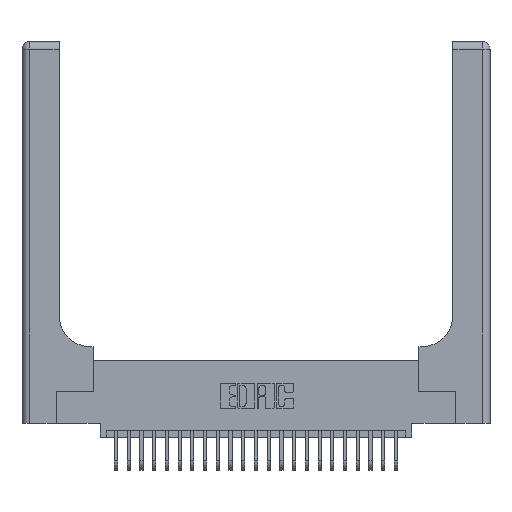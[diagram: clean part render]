
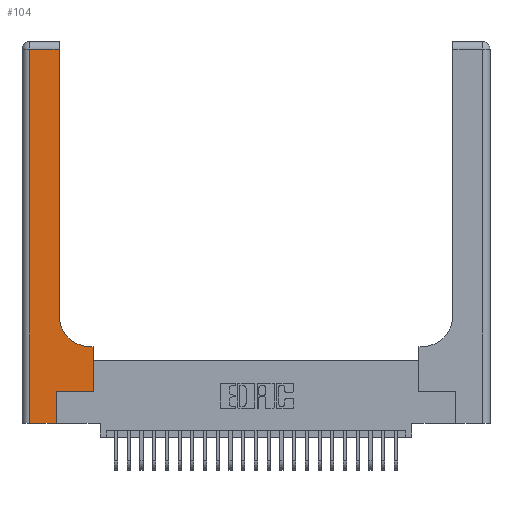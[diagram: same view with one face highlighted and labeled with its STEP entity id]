
A CAD part, top view. The second image highlights one B-rep face of the part: STEP entity #104.
In plain terms, the highlighted planar face has unit normal (0, 0, 1).
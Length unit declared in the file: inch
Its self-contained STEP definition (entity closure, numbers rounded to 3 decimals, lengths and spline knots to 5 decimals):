
#104 = ADVANCED_FACE ( 'NONE', ( #13858 ), #2259, .F. ) ;
#163 = AXIS2_PLACEMENT_3D ( 'NONE', #19622, #6866, #21750 ) ;
#419 = EDGE_CURVE ( 'NONE', #19018, #18135, #22831, .T. ) ;
#757 = ORIENTED_EDGE ( 'NONE', *, *, #15718, .T. ) ;
#1164 = DIRECTION ( 'NONE',  ( 1., 0., 0. ) ) ;
#1200 = EDGE_LOOP ( 'NONE', ( #757, #8010, #6784, #17955, #25926, #12365, #1759, #20742, #6190 ) ) ;
#1759 = ORIENTED_EDGE ( 'NONE', *, *, #11357, .T. ) ;
#1855 = EDGE_CURVE ( 'NONE', #12379, #5063, #2435, .T. ) ;
#2195 = DIRECTION ( 'NONE',  ( -1., 0., 0. ) ) ;
#2230 = DIRECTION ( 'NONE',  ( 0., 0., -1. ) ) ;
#2259 = PLANE ( 'NONE',  #24489 ) ;
#2435 = LINE ( 'NONE', #6089, #13146 ) ;
#2594 = CARTESIAN_POINT ( 'NONE',  ( 0., 3., 0.37 ) ) ;
#2967 = VECTOR ( 'NONE', #24134, 39.37008 ) ;
#3228 = CARTESIAN_POINT ( 'NONE',  ( 0.269, 0., 0.37 ) ) ;
#3309 = VERTEX_POINT ( 'NONE', #18819 ) ;
#4459 = DIRECTION ( 'NONE',  ( -1., 0., 0. ) ) ;
#4768 = EDGE_CURVE ( 'NONE', #19219, #12379, #15252, .T. ) ;
#5063 = VERTEX_POINT ( 'NONE', #24457 ) ;
#5098 = VERTEX_POINT ( 'NONE', #3228 ) ;
#5352 = DIRECTION ( 'NONE',  ( 0., 1., 0. ) ) ;
#5746 = CARTESIAN_POINT ( 'NONE',  ( 0.5585, 0.25, 0.37 ) ) ;
#6009 = LINE ( 'NONE', #24506, #15985 ) ;
#6089 = CARTESIAN_POINT ( 'NONE',  ( 0.06, 3., 0.37 ) ) ;
#6190 = ORIENTED_EDGE ( 'NONE', *, *, #7276, .T. ) ;
#6589 = LINE ( 'NONE', #23222, #21567 ) ;
#6784 = ORIENTED_EDGE ( 'NONE', *, *, #1855, .T. ) ;
#6866 = DIRECTION ( 'NONE',  ( 0., 0., -1. ) ) ;
#7276 = EDGE_CURVE ( 'NONE', #25199, #24083, #23463, .T. ) ;
#8010 = ORIENTED_EDGE ( 'NONE', *, *, #4768, .T. ) ;
#8204 = DIRECTION ( 'NONE',  ( 0., -1., 0. ) ) ;
#9630 = EDGE_CURVE ( 'NONE', #3309, #25199, #11362, .T. ) ;
#10209 = CARTESIAN_POINT ( 'NONE',  ( 0.2915, 0.6, 0.37 ) ) ;
#11357 = EDGE_CURVE ( 'NONE', #18135, #3309, #26075, .T. ) ;
#11362 = LINE ( 'NONE', #10209, #26318 ) ;
#11501 = VECTOR ( 'NONE', #1164, 39.37008 ) ;
#11777 = CARTESIAN_POINT ( 'NONE',  ( 0.5415, 0.6, 0.37 ) ) ;
#12365 = ORIENTED_EDGE ( 'NONE', *, *, #419, .T. ) ;
#12379 = VERTEX_POINT ( 'NONE', #18424 ) ;
#12967 = CARTESIAN_POINT ( 'NONE',  ( 0., 2.94, 0.37 ) ) ;
#13146 = VECTOR ( 'NONE', #8204, 39.37008 ) ;
#13858 = FACE_OUTER_BOUND ( 'NONE', #1200, .T. ) ;
#15252 = LINE ( 'NONE', #12967, #25232 ) ;
#15718 = EDGE_CURVE ( 'NONE', #24083, #19219, #6589, .T. ) ;
#15985 = VECTOR ( 'NONE', #5352, 39.37008 ) ;
#16907 = DIRECTION ( 'NONE',  ( 0., 1., 0. ) ) ;
#17955 = ORIENTED_EDGE ( 'NONE', *, *, #18668, .T. ) ;
#18135 = VERTEX_POINT ( 'NONE', #22239 ) ;
#18424 = CARTESIAN_POINT ( 'NONE',  ( 0.06, 2.94, 0.37 ) ) ;
#18668 = EDGE_CURVE ( 'NONE', #5063, #5098, #19995, .T. ) ;
#18689 = DIRECTION ( 'NONE',  ( -1., 0., 0. ) ) ;
#18799 = EDGE_CURVE ( 'NONE', #5098, #19018, #6009, .T. ) ;
#18819 = CARTESIAN_POINT ( 'NONE',  ( 0.5585, 0.6, 0.37 ) ) ;
#19018 = VERTEX_POINT ( 'NONE', #27194 ) ;
#19219 = VERTEX_POINT ( 'NONE', #23757 ) ;
#19622 = CARTESIAN_POINT ( 'NONE',  ( 0.5415, 0.85, 0.37 ) ) ;
#19995 = LINE ( 'NONE', #22030, #2967 ) ;
#20666 = CARTESIAN_POINT ( 'NONE',  ( 0.2915, 0.85, 0.37 ) ) ;
#20742 = ORIENTED_EDGE ( 'NONE', *, *, #9630, .T. ) ;
#21567 = VECTOR ( 'NONE', #16907, 39.37008 ) ;
#21750 = DIRECTION ( 'NONE',  ( 1., 0., 0. ) ) ;
#22030 = CARTESIAN_POINT ( 'NONE',  ( 0., 0., 0.37 ) ) ;
#22239 = CARTESIAN_POINT ( 'NONE',  ( 0.5585, 0.25, 0.37 ) ) ;
#22776 = DIRECTION ( 'NONE',  ( 0., 1., 0. ) ) ;
#22831 = LINE ( 'NONE', #26690, #11501 ) ;
#23222 = CARTESIAN_POINT ( 'NONE',  ( 0.2915, 3., 0.37 ) ) ;
#23463 = CIRCLE ( 'NONE', #163, 0.25 ) ;
#23757 = CARTESIAN_POINT ( 'NONE',  ( 0.2915, 2.94, 0.37 ) ) ;
#24083 = VERTEX_POINT ( 'NONE', #20666 ) ;
#24134 = DIRECTION ( 'NONE',  ( 1., 0., 0. ) ) ;
#24457 = CARTESIAN_POINT ( 'NONE',  ( 0.06, 0., 0.37 ) ) ;
#24489 = AXIS2_PLACEMENT_3D ( 'NONE', #2594, #2230, #2195 ) ;
#24506 = CARTESIAN_POINT ( 'NONE',  ( 0.269, 0., 0.37 ) ) ;
#25199 = VERTEX_POINT ( 'NONE', #11777 ) ;
#25232 = VECTOR ( 'NONE', #4459, 39.37008 ) ;
#25421 = VECTOR ( 'NONE', #22776, 39.37008 ) ;
#25926 = ORIENTED_EDGE ( 'NONE', *, *, #18799, .T. ) ;
#26075 = LINE ( 'NONE', #5746, #25421 ) ;
#26318 = VECTOR ( 'NONE', #18689, 39.37008 ) ;
#26690 = CARTESIAN_POINT ( 'NONE',  ( 0.269, 0.25, 0.37 ) ) ;
#27194 = CARTESIAN_POINT ( 'NONE',  ( 0.269, 0.25, 0.37 ) ) ;
